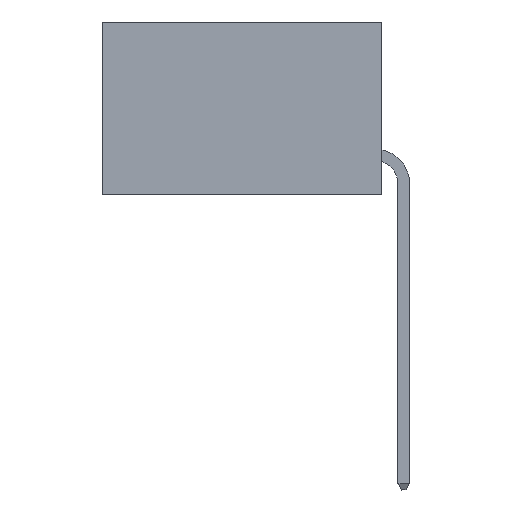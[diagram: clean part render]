
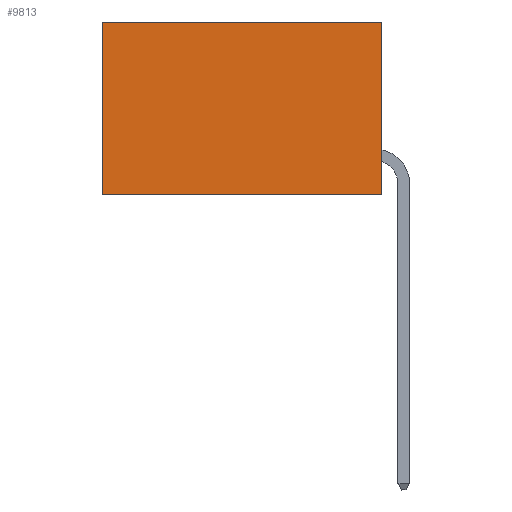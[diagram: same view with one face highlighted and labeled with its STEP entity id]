
A CAD part, left-side view. The second image highlights one B-rep face of the part: STEP entity #9813.
In plain terms, the highlighted planar face has unit normal (-1, 0, 0).
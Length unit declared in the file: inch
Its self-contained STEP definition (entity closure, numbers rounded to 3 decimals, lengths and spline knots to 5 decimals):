
#397 = CARTESIAN_POINT ( 'NONE',  ( 0.2875, 0., 0. ) ) ;
#471 = ORIENTED_EDGE ( 'NONE', *, *, #4222, .F. ) ;
#565 = LINE ( 'NONE', #10301, #4580 ) ;
#772 = FACE_OUTER_BOUND ( 'NONE', #6839, .T. ) ;
#947 = DIRECTION ( 'NONE',  ( 0., 1., 0. ) ) ;
#1002 = CARTESIAN_POINT ( 'NONE',  ( 0.2875, 0., -0.37 ) ) ;
#1261 = DIRECTION ( 'NONE',  ( 0., 0., -1. ) ) ;
#1469 = LINE ( 'NONE', #1002, #2000 ) ;
#1964 = EDGE_CURVE ( 'NONE', #4266, #2638, #565, .T. ) ;
#2000 = VECTOR ( 'NONE', #7752, 39.37008 ) ;
#2212 = LINE ( 'NONE', #10030, #5678 ) ;
#2220 = DIRECTION ( 'NONE',  ( 1., 0., 0. ) ) ;
#2638 = VERTEX_POINT ( 'NONE', #9476 ) ;
#4051 = EDGE_CURVE ( 'NONE', #8772, #7575, #1469, .T. ) ;
#4222 = EDGE_CURVE ( 'NONE', #4266, #8772, #4556, .T. ) ;
#4266 = VERTEX_POINT ( 'NONE', #397 ) ;
#4306 = ORIENTED_EDGE ( 'NONE', *, *, #4051, .F. ) ;
#4556 = LINE ( 'NONE', #4667, #9733 ) ;
#4580 = VECTOR ( 'NONE', #947, 39.37008 ) ;
#4667 = CARTESIAN_POINT ( 'NONE',  ( 0.2875, 0., 0. ) ) ;
#4880 = AXIS2_PLACEMENT_3D ( 'NONE', #5581, #2220, #1261 ) ;
#5141 = EDGE_CURVE ( 'NONE', #2638, #7575, #2212, .T. ) ;
#5581 = CARTESIAN_POINT ( 'NONE',  ( 0.2875, 0., 0. ) ) ;
#5678 = VECTOR ( 'NONE', #8364, 39.37008 ) ;
#6839 = EDGE_LOOP ( 'NONE', ( #7780, #4306, #471, #7617 ) ) ;
#7295 = DIRECTION ( 'NONE',  ( 0., 0., -1. ) ) ;
#7575 = VERTEX_POINT ( 'NONE', #8152 ) ;
#7617 = ORIENTED_EDGE ( 'NONE', *, *, #1964, .T. ) ;
#7752 = DIRECTION ( 'NONE',  ( 0., 1., 0. ) ) ;
#7780 = ORIENTED_EDGE ( 'NONE', *, *, #5141, .T. ) ;
#7946 = CARTESIAN_POINT ( 'NONE',  ( 0.2875, 0., -0.37 ) ) ;
#8152 = CARTESIAN_POINT ( 'NONE',  ( 0.2875, 0.6, -0.37 ) ) ;
#8364 = DIRECTION ( 'NONE',  ( 0., 0., -1. ) ) ;
#8772 = VERTEX_POINT ( 'NONE', #7946 ) ;
#8924 = PLANE ( 'NONE',  #4880 ) ;
#9476 = CARTESIAN_POINT ( 'NONE',  ( 0.2875, 0.6, 0. ) ) ;
#9733 = VECTOR ( 'NONE', #7295, 39.37008 ) ;
#9813 = ADVANCED_FACE ( 'NONE', ( #772 ), #8924, .F. ) ;
#10030 = CARTESIAN_POINT ( 'NONE',  ( 0.2875, 0.6, 0. ) ) ;
#10301 = CARTESIAN_POINT ( 'NONE',  ( 0.2875, 0., 0. ) ) ;
